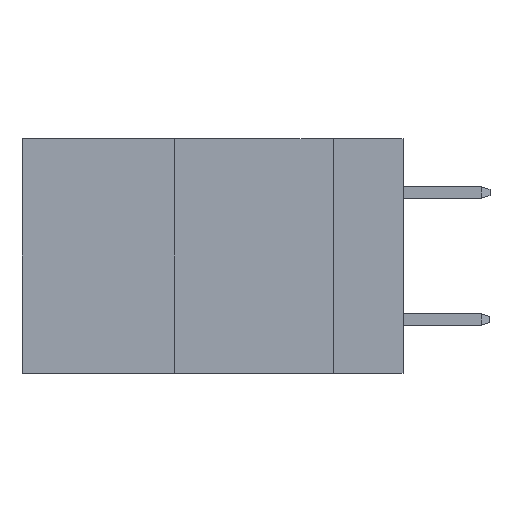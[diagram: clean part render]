
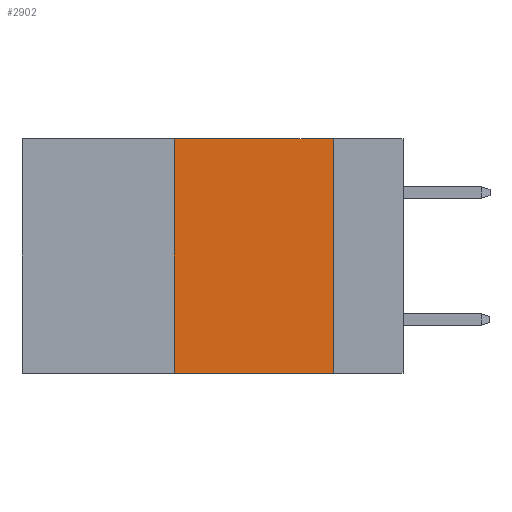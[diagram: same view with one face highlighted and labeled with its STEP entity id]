
A CAD part, left-side view. The second image highlights one B-rep face of the part: STEP entity #2902.
In plain terms, the highlighted planar face has unit normal (-1, 0, 0).
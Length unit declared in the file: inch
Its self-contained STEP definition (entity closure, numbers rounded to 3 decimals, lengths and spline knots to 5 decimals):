
#184 = LINE ( 'NONE', #8158, #7685 ) ;
#314 = EDGE_CURVE ( 'NONE', #7932, #10140, #9460, .T. ) ;
#1275 = CARTESIAN_POINT ( 'NONE',  ( 0., 0.6, 0. ) ) ;
#1292 = VECTOR ( 'NONE', #12271, 39.37008 ) ;
#1410 = CARTESIAN_POINT ( 'NONE',  ( 0., 0.36, 0. ) ) ;
#2222 = VERTEX_POINT ( 'NONE', #8726 ) ;
#2247 = CARTESIAN_POINT ( 'NONE',  ( 0., 0.11, -0.37 ) ) ;
#2359 = FACE_OUTER_BOUND ( 'NONE', #5372, .T. ) ;
#2415 = PLANE ( 'NONE',  #8421 ) ;
#2902 = ADVANCED_FACE ( 'NONE', ( #2359 ), #2415, .F. ) ;
#3134 = DIRECTION ( 'NONE',  ( 0., -1., 0. ) ) ;
#3284 = DIRECTION ( 'NONE',  ( 1., 0., 0. ) ) ;
#3581 = ORIENTED_EDGE ( 'NONE', *, *, #9388, .F. ) ;
#3946 = LINE ( 'NONE', #5705, #11078 ) ;
#4788 = CARTESIAN_POINT ( 'NONE',  ( 0., 0.36, -0.37 ) ) ;
#5372 = EDGE_LOOP ( 'NONE', ( #9176, #3581, #11372, #5879 ) ) ;
#5422 = CARTESIAN_POINT ( 'NONE',  ( 0., 0.6, 0. ) ) ;
#5705 = CARTESIAN_POINT ( 'NONE',  ( 0., 0.11, 0. ) ) ;
#5879 = ORIENTED_EDGE ( 'NONE', *, *, #12535, .T. ) ;
#7347 = LINE ( 'NONE', #1275, #10634 ) ;
#7663 = VERTEX_POINT ( 'NONE', #2247 ) ;
#7685 = VECTOR ( 'NONE', #3134, 39.37008 ) ;
#7932 = VERTEX_POINT ( 'NONE', #4788 ) ;
#8158 = CARTESIAN_POINT ( 'NONE',  ( 0., 0.6, -0.37 ) ) ;
#8159 = CARTESIAN_POINT ( 'NONE',  ( 0., 0.36, 0. ) ) ;
#8421 = AXIS2_PLACEMENT_3D ( 'NONE', #5422, #3284, #9229 ) ;
#8719 = DIRECTION ( 'NONE',  ( 0., 0., -1. ) ) ;
#8726 = CARTESIAN_POINT ( 'NONE',  ( 0., 0.11, 0. ) ) ;
#9176 = ORIENTED_EDGE ( 'NONE', *, *, #9676, .F. ) ;
#9229 = DIRECTION ( 'NONE',  ( 0., 0., -1. ) ) ;
#9388 = EDGE_CURVE ( 'NONE', #10140, #2222, #7347, .T. ) ;
#9460 = LINE ( 'NONE', #1410, #1292 ) ;
#9676 = EDGE_CURVE ( 'NONE', #2222, #7663, #3946, .T. ) ;
#10140 = VERTEX_POINT ( 'NONE', #8159 ) ;
#10634 = VECTOR ( 'NONE', #12065, 39.37008 ) ;
#11078 = VECTOR ( 'NONE', #8719, 39.37008 ) ;
#11372 = ORIENTED_EDGE ( 'NONE', *, *, #314, .F. ) ;
#12065 = DIRECTION ( 'NONE',  ( 0., -1., 0. ) ) ;
#12271 = DIRECTION ( 'NONE',  ( 0., 0., 1. ) ) ;
#12535 = EDGE_CURVE ( 'NONE', #7932, #7663, #184, .T. ) ;
